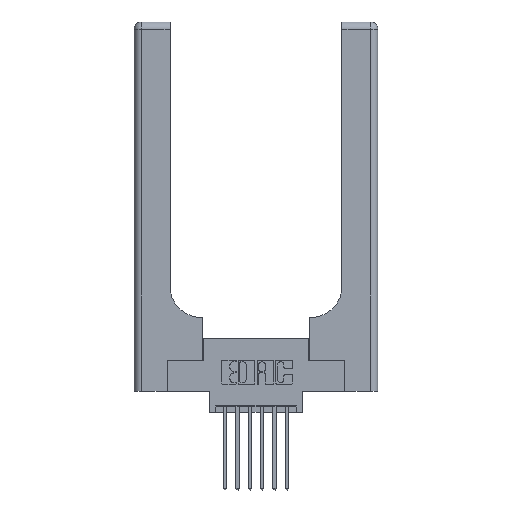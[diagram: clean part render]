
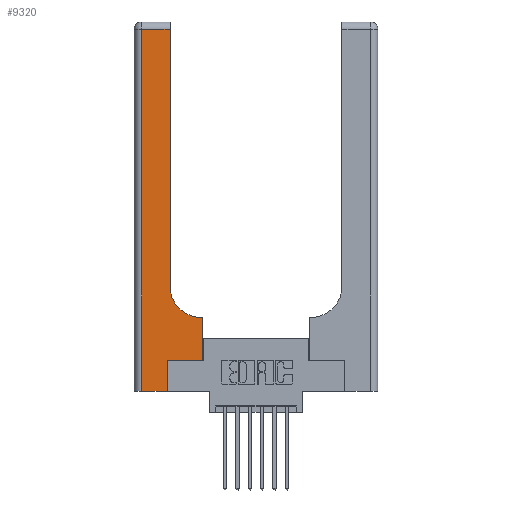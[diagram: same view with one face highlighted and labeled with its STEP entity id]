
A CAD part, top view. The second image highlights one B-rep face of the part: STEP entity #9320.
In plain terms, the highlighted planar face has unit normal (0, 0, 1).
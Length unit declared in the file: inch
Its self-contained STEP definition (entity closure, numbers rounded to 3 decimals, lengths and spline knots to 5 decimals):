
#158 = ORIENTED_EDGE ( 'NONE', *, *, #11158, .T. ) ;
#339 = LINE ( 'NONE', #7078, #12592 ) ;
#360 = ORIENTED_EDGE ( 'NONE', *, *, #10199, .T. ) ;
#413 = VECTOR ( 'NONE', #4391, 39.37008 ) ;
#474 = ORIENTED_EDGE ( 'NONE', *, *, #969, .T. ) ;
#493 = VECTOR ( 'NONE', #11283, 39.37008 ) ;
#526 = VECTOR ( 'NONE', #931, 39.37008 ) ;
#931 = DIRECTION ( 'NONE',  ( 0., 1., 0. ) ) ;
#969 = EDGE_CURVE ( 'NONE', #10554, #13015, #339, .T. ) ;
#1099 = LINE ( 'NONE', #1296, #7274 ) ;
#1296 = CARTESIAN_POINT ( 'NONE',  ( 0.5585, 0.25, 0.37 ) ) ;
#1548 = CARTESIAN_POINT ( 'NONE',  ( 0., 3., 0.37 ) ) ;
#1577 = CARTESIAN_POINT ( 'NONE',  ( 0.5585, 0.25, 0.37 ) ) ;
#1622 = VERTEX_POINT ( 'NONE', #4747 ) ;
#2489 = DIRECTION ( 'NONE',  ( 0., 1., 0. ) ) ;
#2724 = AXIS2_PLACEMENT_3D ( 'NONE', #3541, #11548, #4734 ) ;
#2788 = EDGE_CURVE ( 'NONE', #1622, #9893, #2968, .T. ) ;
#2952 = VERTEX_POINT ( 'NONE', #12855 ) ;
#2968 = LINE ( 'NONE', #11480, #11744 ) ;
#3013 = CARTESIAN_POINT ( 'NONE',  ( 0.2915, 0.6, 0.37 ) ) ;
#3378 = VERTEX_POINT ( 'NONE', #3404 ) ;
#3404 = CARTESIAN_POINT ( 'NONE',  ( 0.06, 2.94, 0.37 ) ) ;
#3512 = ORIENTED_EDGE ( 'NONE', *, *, #2788, .T. ) ;
#3541 = CARTESIAN_POINT ( 'NONE',  ( 0.5415, 0.85, 0.37 ) ) ;
#3938 = LINE ( 'NONE', #13426, #413 ) ;
#4083 = CARTESIAN_POINT ( 'NONE',  ( 0.2915, 3., 0.37 ) ) ;
#4391 = DIRECTION ( 'NONE',  ( 0., -1., 0. ) ) ;
#4629 = ORIENTED_EDGE ( 'NONE', *, *, #10403, .T. ) ;
#4734 = DIRECTION ( 'NONE',  ( 1., 0., 0. ) ) ;
#4747 = CARTESIAN_POINT ( 'NONE',  ( 0.269, 0.25, 0.37 ) ) ;
#4775 = ORIENTED_EDGE ( 'NONE', *, *, #9982, .T. ) ;
#4885 = DIRECTION ( 'NONE',  ( 0., 0., -1. ) ) ;
#5860 = LINE ( 'NONE', #4083, #14895 ) ;
#6386 = LINE ( 'NONE', #11295, #526 ) ;
#6605 = VERTEX_POINT ( 'NONE', #8277 ) ;
#6997 = VERTEX_POINT ( 'NONE', #13755 ) ;
#7055 = EDGE_LOOP ( 'NONE', ( #4775, #158, #14200, #474, #360, #3512, #4629, #8021, #7836 ) ) ;
#7074 = DIRECTION ( 'NONE',  ( 1., 0., 0. ) ) ;
#7078 = CARTESIAN_POINT ( 'NONE',  ( 0., 0., 0.37 ) ) ;
#7274 = VECTOR ( 'NONE', #2489, 39.37008 ) ;
#7693 = VERTEX_POINT ( 'NONE', #9288 ) ;
#7836 = ORIENTED_EDGE ( 'NONE', *, *, #13228, .T. ) ;
#8021 = ORIENTED_EDGE ( 'NONE', *, *, #8384, .T. ) ;
#8100 = DIRECTION ( 'NONE',  ( 1., 0., 0. ) ) ;
#8277 = CARTESIAN_POINT ( 'NONE',  ( 0.5415, 0.6, 0.37 ) ) ;
#8384 = EDGE_CURVE ( 'NONE', #6997, #6605, #11939, .T. ) ;
#8456 = PLANE ( 'NONE',  #12275 ) ;
#8737 = FACE_OUTER_BOUND ( 'NONE', #7055, .T. ) ;
#8858 = CARTESIAN_POINT ( 'NONE',  ( 0.269, 0., 0.37 ) ) ;
#9288 = CARTESIAN_POINT ( 'NONE',  ( 0.2915, 2.94, 0.37 ) ) ;
#9320 = ADVANCED_FACE ( 'NONE', ( #8737 ), #8456, .F. ) ;
#9743 = LINE ( 'NONE', #10150, #493 ) ;
#9869 = DIRECTION ( 'NONE',  ( -1., 0., 0. ) ) ;
#9893 = VERTEX_POINT ( 'NONE', #1577 ) ;
#9982 = EDGE_CURVE ( 'NONE', #2952, #7693, #5860, .T. ) ;
#10150 = CARTESIAN_POINT ( 'NONE',  ( 0., 2.94, 0.37 ) ) ;
#10199 = EDGE_CURVE ( 'NONE', #13015, #1622, #6386, .T. ) ;
#10403 = EDGE_CURVE ( 'NONE', #9893, #6997, #1099, .T. ) ;
#10554 = VERTEX_POINT ( 'NONE', #11115 ) ;
#10740 = DIRECTION ( 'NONE',  ( -1., 0., 0. ) ) ;
#10927 = CIRCLE ( 'NONE', #2724, 0.25 ) ;
#11115 = CARTESIAN_POINT ( 'NONE',  ( 0.06, 0., 0.37 ) ) ;
#11158 = EDGE_CURVE ( 'NONE', #7693, #3378, #9743, .T. ) ;
#11221 = VECTOR ( 'NONE', #9869, 39.37008 ) ;
#11283 = DIRECTION ( 'NONE',  ( -1., 0., 0. ) ) ;
#11295 = CARTESIAN_POINT ( 'NONE',  ( 0.269, 0., 0.37 ) ) ;
#11480 = CARTESIAN_POINT ( 'NONE',  ( 0.269, 0.25, 0.37 ) ) ;
#11548 = DIRECTION ( 'NONE',  ( 0., 0., -1. ) ) ;
#11744 = VECTOR ( 'NONE', #8100, 39.37008 ) ;
#11939 = LINE ( 'NONE', #3013, #11221 ) ;
#12039 = DIRECTION ( 'NONE',  ( 0., 1., 0. ) ) ;
#12275 = AXIS2_PLACEMENT_3D ( 'NONE', #1548, #4885, #10740 ) ;
#12592 = VECTOR ( 'NONE', #7074, 39.37008 ) ;
#12855 = CARTESIAN_POINT ( 'NONE',  ( 0.2915, 0.85, 0.37 ) ) ;
#13015 = VERTEX_POINT ( 'NONE', #8858 ) ;
#13228 = EDGE_CURVE ( 'NONE', #6605, #2952, #10927, .T. ) ;
#13426 = CARTESIAN_POINT ( 'NONE',  ( 0.06, 3., 0.37 ) ) ;
#13755 = CARTESIAN_POINT ( 'NONE',  ( 0.5585, 0.6, 0.37 ) ) ;
#14043 = EDGE_CURVE ( 'NONE', #3378, #10554, #3938, .T. ) ;
#14200 = ORIENTED_EDGE ( 'NONE', *, *, #14043, .T. ) ;
#14895 = VECTOR ( 'NONE', #12039, 39.37008 ) ;
